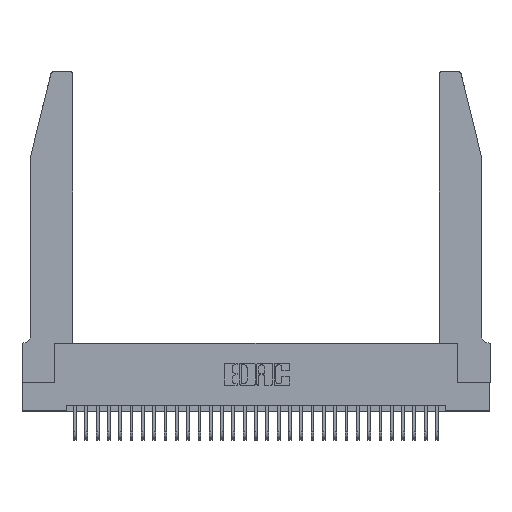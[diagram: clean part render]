
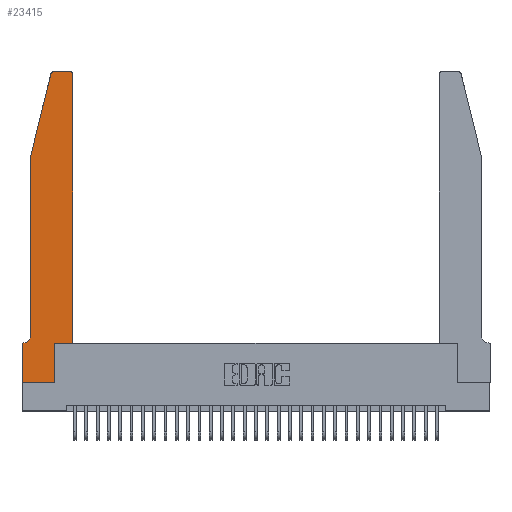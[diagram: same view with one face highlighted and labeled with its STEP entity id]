
A CAD part, top view. The second image highlights one B-rep face of the part: STEP entity #23415.
In plain terms, the highlighted planar face has unit normal (0, 0, 1).
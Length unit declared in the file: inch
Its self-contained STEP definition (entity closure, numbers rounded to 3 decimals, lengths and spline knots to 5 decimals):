
#506 = AXIS2_PLACEMENT_3D ( 'NONE', #2124, #18850, #4565 ) ;
#517 = CARTESIAN_POINT ( 'NONE',  ( 0., 0., 0.37 ) ) ;
#1145 = DIRECTION ( 'NONE',  ( 1., 0., 0. ) ) ;
#1190 = DIRECTION ( 'NONE',  ( 1., 0., 0. ) ) ;
#1625 = VECTOR ( 'NONE', #29071, 39.37008 ) ;
#1909 = ORIENTED_EDGE ( 'NONE', *, *, #26012, .T. ) ;
#1967 = LINE ( 'NONE', #8049, #26570 ) ;
#1969 = CARTESIAN_POINT ( 'NONE',  ( 0.4205, 2.75, 0.37 ) ) ;
#2031 = EDGE_CURVE ( 'NONE', #25781, #5166, #8415, .T. ) ;
#2038 = VECTOR ( 'NONE', #7595, 39.37008 ) ;
#2112 = VECTOR ( 'NONE', #2323, 39.37008 ) ;
#2124 = CARTESIAN_POINT ( 'NONE',  ( 0.0055, 0.42, 0.37 ) ) ;
#2323 = DIRECTION ( 'NONE',  ( -1., 0., 0. ) ) ;
#2457 = CARTESIAN_POINT ( 'NONE',  ( 0.2865, 0.35, 0.37 ) ) ;
#2752 = CARTESIAN_POINT ( 'NONE',  ( 0., 0., 0.37 ) ) ;
#2804 = DIRECTION ( 'NONE',  ( 0., 1., 0. ) ) ;
#2867 = VERTEX_POINT ( 'NONE', #27682 ) ;
#2929 = CARTESIAN_POINT ( 'NONE',  ( 0.25487, 2.72718, 0.37 ) ) ;
#3080 = VECTOR ( 'NONE', #17655, 39.37008 ) ;
#3335 = CARTESIAN_POINT ( 'NONE',  ( 0.284, 2.75, 0.37 ) ) ;
#3562 = AXIS2_PLACEMENT_3D ( 'NONE', #29758, #15543, #1190 ) ;
#3588 = VECTOR ( 'NONE', #6393, 39.37008 ) ;
#4069 = VERTEX_POINT ( 'NONE', #22011 ) ;
#4511 = LINE ( 'NONE', #11713, #11593 ) ;
#4565 = DIRECTION ( 'NONE',  ( -1., 0., 0. ) ) ;
#4668 = CARTESIAN_POINT ( 'NONE',  ( 0.0755, 0.35, 0.37 ) ) ;
#5166 = VERTEX_POINT ( 'NONE', #7076 ) ;
#6393 = DIRECTION ( 'NONE',  ( -1., 0., 0. ) ) ;
#7076 = CARTESIAN_POINT ( 'NONE',  ( 0., 0., 0.37 ) ) ;
#7595 = DIRECTION ( 'NONE',  ( 0., -1., 0. ) ) ;
#7678 = CARTESIAN_POINT ( 'NONE',  ( 0.2865, 0., 0.37 ) ) ;
#8008 = CARTESIAN_POINT ( 'NONE',  ( 0.0755, 0.42, 0.37 ) ) ;
#8025 = LINE ( 'NONE', #517, #1625 ) ;
#8049 = CARTESIAN_POINT ( 'NONE',  ( 0.0755, 2., 0.37 ) ) ;
#8415 = LINE ( 'NONE', #2752, #2038 ) ;
#8473 = CARTESIAN_POINT ( 'NONE',  ( 0.4505, 0.35, 0.37 ) ) ;
#8485 = LINE ( 'NONE', #4668, #2112 ) ;
#8596 = CARTESIAN_POINT ( 'NONE',  ( 0.0055, 0.35, 0.37 ) ) ;
#8674 = CARTESIAN_POINT ( 'NONE',  ( 0.2605, 2.75, 0.37 ) ) ;
#9005 = ORIENTED_EDGE ( 'NONE', *, *, #15882, .T. ) ;
#9131 = EDGE_CURVE ( 'NONE', #2867, #13849, #9547, .T. ) ;
#9450 = LINE ( 'NONE', #24683, #3080 ) ;
#9547 = CIRCLE ( 'NONE', #21730, 0.03 ) ;
#9676 = ORIENTED_EDGE ( 'NONE', *, *, #26951, .T. ) ;
#9829 = EDGE_CURVE ( 'NONE', #30056, #2867, #16575, .T. ) ;
#9954 = LINE ( 'NONE', #8674, #3588 ) ;
#9992 = CIRCLE ( 'NONE', #506, 0.07 ) ;
#10237 = VECTOR ( 'NONE', #15675, 39.37008 ) ;
#10364 = ORIENTED_EDGE ( 'NONE', *, *, #23541, .T. ) ;
#11593 = VECTOR ( 'NONE', #28331, 39.37008 ) ;
#11713 = CARTESIAN_POINT ( 'NONE',  ( 0.4505, 0.35, 0.37 ) ) ;
#12819 = DIRECTION ( 'NONE',  ( 0., -1., 0. ) ) ;
#13849 = VERTEX_POINT ( 'NONE', #1969 ) ;
#14053 = EDGE_CURVE ( 'NONE', #20119, #27331, #26362, .T. ) ;
#14483 = VECTOR ( 'NONE', #2804, 39.37008 ) ;
#14587 = FACE_OUTER_BOUND ( 'NONE', #18274, .T. ) ;
#14924 = AXIS2_PLACEMENT_3D ( 'NONE', #27709, #30114, #15910 ) ;
#15498 = DIRECTION ( 'NONE',  ( 0., 0., 1. ) ) ;
#15543 = DIRECTION ( 'NONE',  ( 0., 0., 1. ) ) ;
#15565 = ORIENTED_EDGE ( 'NONE', *, *, #9131, .T. ) ;
#15675 = DIRECTION ( 'NONE',  ( 0., 1., 0. ) ) ;
#15700 = ORIENTED_EDGE ( 'NONE', *, *, #28763, .T. ) ;
#15873 = CARTESIAN_POINT ( 'NONE',  ( 0., 0.35, 0.37 ) ) ;
#15882 = EDGE_CURVE ( 'NONE', #5166, #20119, #8025, .T. ) ;
#15910 = DIRECTION ( 'NONE',  ( 1., 0., 0. ) ) ;
#16539 = EDGE_CURVE ( 'NONE', #4069, #19582, #1967, .T. ) ;
#16575 = LINE ( 'NONE', #8473, #10237 ) ;
#17127 = CARTESIAN_POINT ( 'NONE',  ( 0.2865, 0.35, 0.37 ) ) ;
#17655 = DIRECTION ( 'NONE',  ( -0.239, -0.971, 0. ) ) ;
#18274 = EDGE_LOOP ( 'NONE', ( #29187, #9676, #15700, #18982, #1909, #29764, #28349, #9005, #27683, #10364, #22038, #15565 ) ) ;
#18850 = DIRECTION ( 'NONE',  ( 0., 0., -1. ) ) ;
#18982 = ORIENTED_EDGE ( 'NONE', *, *, #16539, .T. ) ;
#19582 = VERTEX_POINT ( 'NONE', #8008 ) ;
#20119 = VERTEX_POINT ( 'NONE', #7678 ) ;
#20598 = PLANE ( 'NONE',  #14924 ) ;
#21730 = AXIS2_PLACEMENT_3D ( 'NONE', #29715, #15498, #1145 ) ;
#22011 = CARTESIAN_POINT ( 'NONE',  ( 0.0755, 2., 0.37 ) ) ;
#22038 = ORIENTED_EDGE ( 'NONE', *, *, #9829, .T. ) ;
#23305 = CIRCLE ( 'NONE', #3562, 0.03 ) ;
#23415 = ADVANCED_FACE ( 'NONE', ( #14587 ), #20598, .T. ) ;
#23541 = EDGE_CURVE ( 'NONE', #27331, #30056, #4511, .T. ) ;
#23776 = VERTEX_POINT ( 'NONE', #2929 ) ;
#24106 = CARTESIAN_POINT ( 'NONE',  ( 0.4505, 0.35, 0.37 ) ) ;
#24683 = CARTESIAN_POINT ( 'NONE',  ( 0.0755, 2., 0.37 ) ) ;
#25777 = EDGE_CURVE ( 'NONE', #13849, #26905, #9954, .T. ) ;
#25781 = VERTEX_POINT ( 'NONE', #15873 ) ;
#26012 = EDGE_CURVE ( 'NONE', #19582, #28306, #9992, .T. ) ;
#26074 = EDGE_CURVE ( 'NONE', #28306, #25781, #8485, .T. ) ;
#26362 = LINE ( 'NONE', #17127, #14483 ) ;
#26570 = VECTOR ( 'NONE', #12819, 39.37008 ) ;
#26905 = VERTEX_POINT ( 'NONE', #3335 ) ;
#26951 = EDGE_CURVE ( 'NONE', #26905, #23776, #23305, .T. ) ;
#27331 = VERTEX_POINT ( 'NONE', #2457 ) ;
#27682 = CARTESIAN_POINT ( 'NONE',  ( 0.4505, 2.72, 0.37 ) ) ;
#27683 = ORIENTED_EDGE ( 'NONE', *, *, #14053, .T. ) ;
#27709 = CARTESIAN_POINT ( 'NONE',  ( 0., 0.35, 0.37 ) ) ;
#28306 = VERTEX_POINT ( 'NONE', #8596 ) ;
#28331 = DIRECTION ( 'NONE',  ( 1., 0., 0. ) ) ;
#28349 = ORIENTED_EDGE ( 'NONE', *, *, #2031, .T. ) ;
#28763 = EDGE_CURVE ( 'NONE', #23776, #4069, #9450, .T. ) ;
#29071 = DIRECTION ( 'NONE',  ( 1., 0., 0. ) ) ;
#29187 = ORIENTED_EDGE ( 'NONE', *, *, #25777, .T. ) ;
#29715 = CARTESIAN_POINT ( 'NONE',  ( 0.4205, 2.72, 0.37 ) ) ;
#29758 = CARTESIAN_POINT ( 'NONE',  ( 0.284, 2.72, 0.37 ) ) ;
#29764 = ORIENTED_EDGE ( 'NONE', *, *, #26074, .T. ) ;
#30056 = VERTEX_POINT ( 'NONE', #24106 ) ;
#30114 = DIRECTION ( 'NONE',  ( 0., 0., 1. ) ) ;
